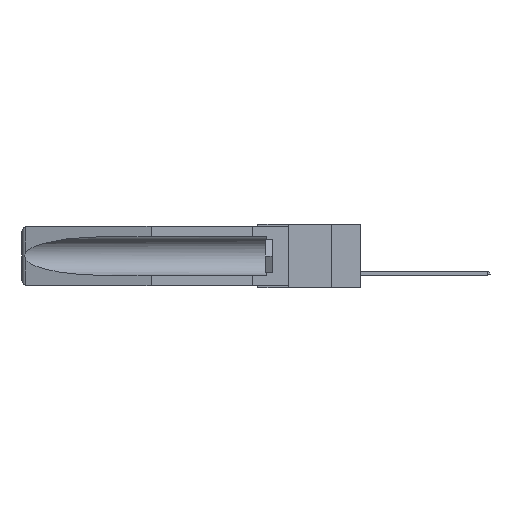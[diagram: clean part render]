
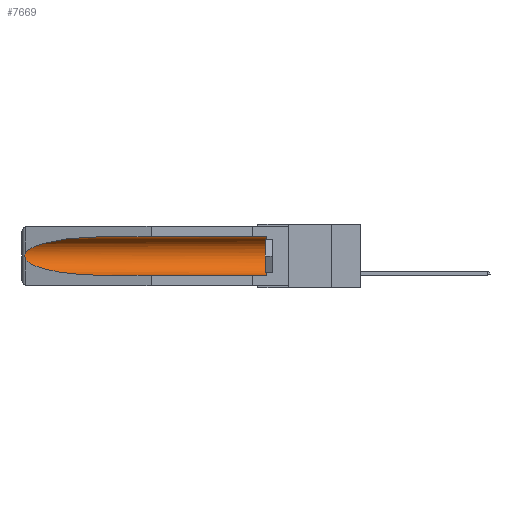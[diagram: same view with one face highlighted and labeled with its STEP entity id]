
A CAD part, left-side view. The second image highlights one B-rep face of the part: STEP entity #7669.
In plain terms, the highlighted cylindrical face has radius 2.857 mm (diameter 5.715 mm), a partial arc.
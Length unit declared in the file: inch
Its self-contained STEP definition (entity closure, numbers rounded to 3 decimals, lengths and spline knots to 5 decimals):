
#253 = CARTESIAN_POINT ( 'NONE',  ( 0.2673, 1.53269, -0.17917 ) ) ;
#416 = ORIENTED_EDGE ( 'NONE', *, *, #696, .F. ) ;
#451 = CARTESIAN_POINT ( 'NONE',  ( 0.26537, 1.52718, -0.14972 ) ) ;
#606 = EDGE_CURVE ( 'NONE', #9600, #30283, #6787, .T. ) ;
#672 = VECTOR ( 'NONE', #22774, 39.37008 ) ;
#696 = EDGE_CURVE ( 'NONE', #12843, #6164, #9854, .T. ) ;
#1130 = ORIENTED_EDGE ( 'NONE', *, *, #21203, .T. ) ;
#1204 = ORIENTED_EDGE ( 'NONE', *, *, #11384, .T. ) ;
#1352 = CARTESIAN_POINT ( 'NONE',  ( 0.155, -0.30754, -0.059 ) ) ;
#1611 = ORIENTED_EDGE ( 'NONE', *, *, #5190, .T. ) ;
#2266 = CARTESIAN_POINT ( 'NONE',  ( 0.155, 1.07973, -0.059 ) ) ;
#2902 = DIRECTION ( 'NONE',  ( 0., -1., 0. ) ) ;
#2911 = CARTESIAN_POINT ( 'NONE',  ( 0.26655, 1.53094, -0.18657 ) ) ;
#3582 = CARTESIAN_POINT ( 'NONE',  ( 0.155, -0.30754, -0.284 ) ) ;
#4331 = CARTESIAN_POINT ( 'NONE',  ( 0.26537, 1.52718, -0.19328 ) ) ;
#5161 = CARTESIAN_POINT ( 'NONE',  ( 0.26654, 1.53092, -0.15636 ) ) ;
#5190 = EDGE_CURVE ( 'NONE', #12166, #6164, #25551, .T. ) ;
#6164 = VERTEX_POINT ( 'NONE', #13292 ) ;
#6787 =( BOUNDED_CURVE ( )  B_SPLINE_CURVE ( 3, ( #2266, #8927, #9239, #9128 ),
 .UNSPECIFIED., .F., .F. ) 
 B_SPLINE_CURVE_WITH_KNOTS ( ( 4, 4 ),
 ( 4.71239, 6.08839 ),
 .UNSPECIFIED. ) 
 CURVE ( )  GEOMETRIC_REPRESENTATION_ITEM ( )  RATIONAL_B_SPLINE_CURVE ( ( 1., 0.848, 0.848, 1. ) ) 
 REPRESENTATION_ITEM ( '' )  );
#7506 = CARTESIAN_POINT ( 'NONE',  ( 0.26597, 1.5296, -0.19026 ) ) ;
#7669 = ADVANCED_FACE ( 'NONE', ( #9003 ), #25633, .F. ) ;
#8927 = CARTESIAN_POINT ( 'NONE',  ( 0.21114, 1.30732, -0.059 ) ) ;
#9003 = FACE_OUTER_BOUND ( 'NONE', #16292, .T. ) ;
#9128 = CARTESIAN_POINT ( 'NONE',  ( 0.26537, 1.52718, -0.14972 ) ) ;
#9239 = CARTESIAN_POINT ( 'NONE',  ( 0.25451, 1.48313, -0.09465 ) ) ;
#9600 = VERTEX_POINT ( 'NONE', #20175 ) ;
#9854 = LINE ( 'NONE', #3582, #23159 ) ;
#10155 = CARTESIAN_POINT ( 'NONE',  ( 0.26537, 1.52718, -0.14972 ) ) ;
#11068 = AXIS2_PLACEMENT_3D ( 'NONE', #19702, #12536, #14591 ) ;
#11384 = EDGE_CURVE ( 'NONE', #13978, #9600, #12782, .T. ) ;
#11553 = ORIENTED_EDGE ( 'NONE', *, *, #22157, .T. ) ;
#11835 = CARTESIAN_POINT ( 'NONE',  ( 0.26537, 1.52718, -0.19328 ) ) ;
#12166 = VERTEX_POINT ( 'NONE', #21676 ) ;
#12536 = DIRECTION ( 'NONE',  ( 0., 1., 0. ) ) ;
#12782 = LINE ( 'NONE', #1352, #672 ) ;
#12843 = VERTEX_POINT ( 'NONE', #14376 ) ;
#13292 = CARTESIAN_POINT ( 'NONE',  ( 0.155, 1.07973, -0.284 ) ) ;
#13775 = CARTESIAN_POINT ( 'NONE',  ( 0.21114, 1.30732, -0.284 ) ) ;
#13978 = VERTEX_POINT ( 'NONE', #16641 ) ;
#14269 = CIRCLE ( 'NONE', #23598, 0.1125 ) ;
#14376 = CARTESIAN_POINT ( 'NONE',  ( 0.155, 0.126, -0.284 ) ) ;
#14591 = DIRECTION ( 'NONE',  ( 0., 0., 1. ) ) ;
#15050 = B_SPLINE_CURVE_WITH_KNOTS ( 'NONE', 3,
 ( #451, #16994, #5161, #26027, #21665, #28477, #253, #2911, #7506, #11835 ),
 .UNSPECIFIED., .F., .F.,
 ( 4, 2, 2, 2, 4 ),
 ( 0., 0.00029, 0.00058, 0.00087, 0.00117 ),
 .UNSPECIFIED. ) ;
#16292 = EDGE_LOOP ( 'NONE', ( #28615, #11553, #1611, #416, #1130, #1204 ) ) ;
#16641 = CARTESIAN_POINT ( 'NONE',  ( 0.155, 0.126, -0.059 ) ) ;
#16994 = CARTESIAN_POINT ( 'NONE',  ( 0.26597, 1.52961, -0.15275 ) ) ;
#17382 = CARTESIAN_POINT ( 'NONE',  ( 0.155, 0.126, -0.1715 ) ) ;
#19102 = DIRECTION ( 'NONE',  ( 0., 1., 0. ) ) ;
#19702 = CARTESIAN_POINT ( 'NONE',  ( 0.155, -0.30754, -0.1715 ) ) ;
#20175 = CARTESIAN_POINT ( 'NONE',  ( 0.155, 1.07973, -0.059 ) ) ;
#21203 = EDGE_CURVE ( 'NONE', #12843, #13978, #14269, .T. ) ;
#21665 = CARTESIAN_POINT ( 'NONE',  ( 0.2675, 1.53308, -0.16763 ) ) ;
#21676 = CARTESIAN_POINT ( 'NONE',  ( 0.26537, 1.52718, -0.19328 ) ) ;
#22157 = EDGE_CURVE ( 'NONE', #30283, #12166, #15050, .T. ) ;
#22774 = DIRECTION ( 'NONE',  ( 0., 1., 0. ) ) ;
#23159 = VECTOR ( 'NONE', #19102, 39.37008 ) ;
#23206 = CARTESIAN_POINT ( 'NONE',  ( 0.25451, 1.48313, -0.24835 ) ) ;
#23598 = AXIS2_PLACEMENT_3D ( 'NONE', #17382, #2902, #26712 ) ;
#25551 =( BOUNDED_CURVE ( )  B_SPLINE_CURVE ( 3, ( #4331, #23206, #13775, #30337 ),
 .UNSPECIFIED., .F., .F. ) 
 B_SPLINE_CURVE_WITH_KNOTS ( ( 4, 4 ),
 ( 0.1948, 1.5708 ),
 .UNSPECIFIED. ) 
 CURVE ( )  GEOMETRIC_REPRESENTATION_ITEM ( )  RATIONAL_B_SPLINE_CURVE ( ( 1., 0.848, 0.848, 1. ) ) 
 REPRESENTATION_ITEM ( '' )  );
#25633 = CYLINDRICAL_SURFACE ( 'NONE', #11068, 0.1125 ) ;
#26027 = CARTESIAN_POINT ( 'NONE',  ( 0.2673, 1.5327, -0.16383 ) ) ;
#26712 = DIRECTION ( 'NONE',  ( 0., 0., 1. ) ) ;
#28477 = CARTESIAN_POINT ( 'NONE',  ( 0.2675, 1.53308, -0.17534 ) ) ;
#28615 = ORIENTED_EDGE ( 'NONE', *, *, #606, .T. ) ;
#30283 = VERTEX_POINT ( 'NONE', #10155 ) ;
#30337 = CARTESIAN_POINT ( 'NONE',  ( 0.155, 1.07973, -0.284 ) ) ;
